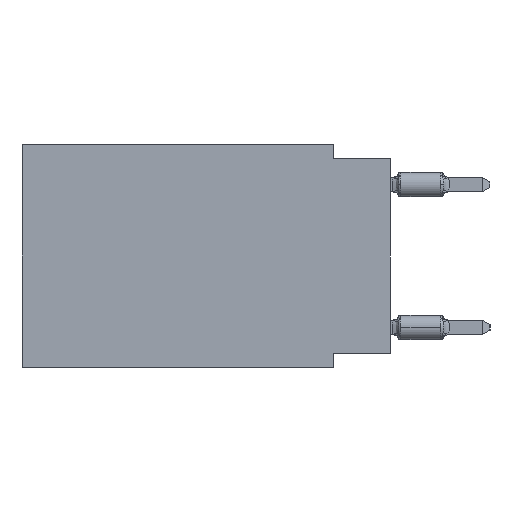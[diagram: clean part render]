
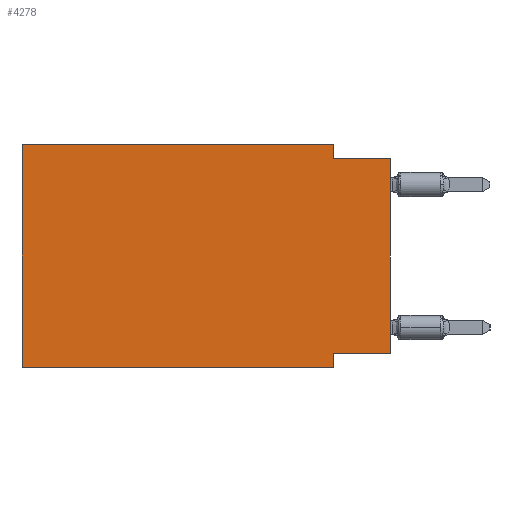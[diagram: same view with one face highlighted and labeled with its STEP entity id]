
A CAD part, left-side view. The second image highlights one B-rep face of the part: STEP entity #4278.
In plain terms, the highlighted planar face has unit normal (-1, 0, 0).
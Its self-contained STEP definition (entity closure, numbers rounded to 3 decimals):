
#985 = ORIENTED_EDGE ( 'NONE', *, *, #28947, .F. ) ;
#1154 = EDGE_LOOP ( 'NONE', ( #10977, #18981, #5436, #28448, #25593, #23650, #985, #26684 ) ) ;
#1196 = CARTESIAN_POINT ( 'NONE',  ( 0., 2.54, -9.906 ) ) ;
#1286 = CARTESIAN_POINT ( 'NONE',  ( 0., 16.383, -9.906 ) ) ;
#1463 = CARTESIAN_POINT ( 'NONE',  ( 0., 16.383, 0. ) ) ;
#1656 = VECTOR ( 'NONE', #13759, 1000. ) ;
#1967 = VECTOR ( 'NONE', #5680, 1000. ) ;
#2509 = DIRECTION ( 'NONE',  ( 0., 0., -1. ) ) ;
#3609 = CARTESIAN_POINT ( 'NONE',  ( 0., 0., -9.271 ) ) ;
#3944 = VECTOR ( 'NONE', #33596, 1000. ) ;
#4278 = ADVANCED_FACE ( 'NONE', ( #9223 ), #11627, .F. ) ;
#4408 = DIRECTION ( 'NONE',  ( 1., 0., 0. ) ) ;
#4751 = EDGE_CURVE ( 'NONE', #20582, #11324, #27562, .T. ) ;
#4881 = DIRECTION ( 'NONE',  ( 0., 0., 1. ) ) ;
#4996 = EDGE_CURVE ( 'NONE', #25059, #18312, #26329, .T. ) ;
#5231 = CARTESIAN_POINT ( 'NONE',  ( 0., 0., -0.635 ) ) ;
#5436 = ORIENTED_EDGE ( 'NONE', *, *, #22826, .F. ) ;
#5680 = DIRECTION ( 'NONE',  ( 0., 1., 0. ) ) ;
#5883 = CARTESIAN_POINT ( 'NONE',  ( 0., 2.54, 0. ) ) ;
#6799 = CARTESIAN_POINT ( 'NONE',  ( 0., 16.383, 0. ) ) ;
#6840 = VECTOR ( 'NONE', #4881, 1000. ) ;
#6885 = VECTOR ( 'NONE', #2509, 1000. ) ;
#9223 = FACE_OUTER_BOUND ( 'NONE', #1154, .T. ) ;
#9422 = VERTEX_POINT ( 'NONE', #19474 ) ;
#10977 = ORIENTED_EDGE ( 'NONE', *, *, #13145, .T. ) ;
#11205 = DIRECTION ( 'NONE',  ( 0., -1., 0. ) ) ;
#11324 = VERTEX_POINT ( 'NONE', #1196 ) ;
#11627 = PLANE ( 'NONE',  #26906 ) ;
#11898 = CARTESIAN_POINT ( 'NONE',  ( 0., 2.54, -9.271 ) ) ;
#12693 = CARTESIAN_POINT ( 'NONE',  ( 0., 2.54, 0. ) ) ;
#13145 = EDGE_CURVE ( 'NONE', #29562, #22321, #30998, .T. ) ;
#13729 = LINE ( 'NONE', #29226, #1967 ) ;
#13759 = DIRECTION ( 'NONE',  ( 0., 0., -1. ) ) ;
#13931 = LINE ( 'NONE', #5883, #1656 ) ;
#14169 = DIRECTION ( 'NONE',  ( 0., 0., 1. ) ) ;
#14284 = EDGE_CURVE ( 'NONE', #20582, #25059, #16570, .T. ) ;
#15331 = CARTESIAN_POINT ( 'NONE',  ( 0., 0., 0. ) ) ;
#16570 = LINE ( 'NONE', #1463, #17287 ) ;
#17269 = CARTESIAN_POINT ( 'NONE',  ( 0., 16.383, 0. ) ) ;
#17287 = VECTOR ( 'NONE', #14169, 1000. ) ;
#18312 = VERTEX_POINT ( 'NONE', #12693 ) ;
#18423 = CARTESIAN_POINT ( 'NONE',  ( 0., 16.383, 0. ) ) ;
#18981 = ORIENTED_EDGE ( 'NONE', *, *, #33812, .F. ) ;
#19474 = CARTESIAN_POINT ( 'NONE',  ( 0., 2.54, -0.635 ) ) ;
#20522 = CARTESIAN_POINT ( 'NONE',  ( 0., 0., -0.635 ) ) ;
#20582 = VERTEX_POINT ( 'NONE', #32553 ) ;
#20803 = VECTOR ( 'NONE', #11205, 1000. ) ;
#22321 = VERTEX_POINT ( 'NONE', #20522 ) ;
#22599 = DIRECTION ( 'NONE',  ( 0., 0., -1. ) ) ;
#22826 = EDGE_CURVE ( 'NONE', #18312, #9422, #13931, .T. ) ;
#23088 = LINE ( 'NONE', #5231, #3944 ) ;
#23650 = ORIENTED_EDGE ( 'NONE', *, *, #4751, .T. ) ;
#24979 = DIRECTION ( 'NONE',  ( 0., -1., 0. ) ) ;
#25059 = VERTEX_POINT ( 'NONE', #6799 ) ;
#25593 = ORIENTED_EDGE ( 'NONE', *, *, #14284, .F. ) ;
#26028 = CARTESIAN_POINT ( 'NONE',  ( 0., 2.54, -9.906 ) ) ;
#26329 = LINE ( 'NONE', #18423, #20803 ) ;
#26684 = ORIENTED_EDGE ( 'NONE', *, *, #29374, .F. ) ;
#26906 = AXIS2_PLACEMENT_3D ( 'NONE', #17269, #4408, #22599 ) ;
#27562 = LINE ( 'NONE', #1286, #29049 ) ;
#28448 = ORIENTED_EDGE ( 'NONE', *, *, #4996, .F. ) ;
#28947 = EDGE_CURVE ( 'NONE', #32928, #11324, #31383, .T. ) ;
#29049 = VECTOR ( 'NONE', #24979, 1000. ) ;
#29226 = CARTESIAN_POINT ( 'NONE',  ( 0., 0., -9.271 ) ) ;
#29374 = EDGE_CURVE ( 'NONE', #29562, #32928, #13729, .T. ) ;
#29562 = VERTEX_POINT ( 'NONE', #3609 ) ;
#30998 = LINE ( 'NONE', #15331, #6840 ) ;
#31383 = LINE ( 'NONE', #26028, #6885 ) ;
#32553 = CARTESIAN_POINT ( 'NONE',  ( 0., 16.383, -9.906 ) ) ;
#32928 = VERTEX_POINT ( 'NONE', #11898 ) ;
#33596 = DIRECTION ( 'NONE',  ( 0., -1., 0. ) ) ;
#33812 = EDGE_CURVE ( 'NONE', #9422, #22321, #23088, .T. ) ;
